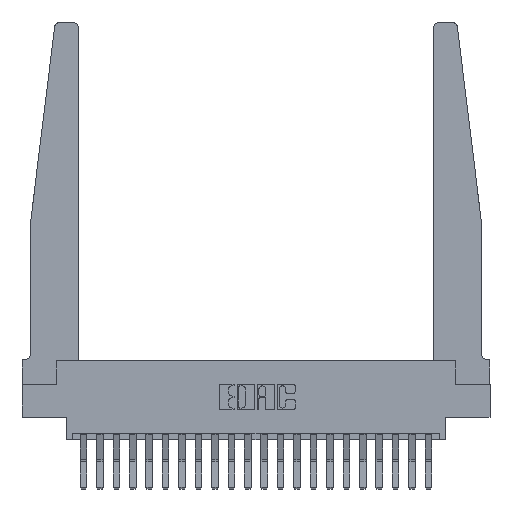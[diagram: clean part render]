
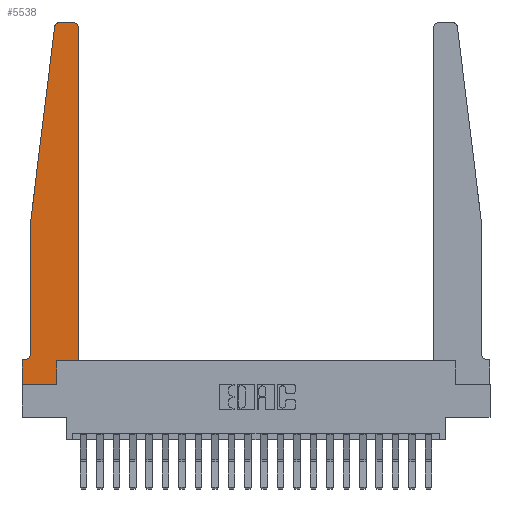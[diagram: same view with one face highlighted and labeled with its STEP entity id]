
A CAD part, top view. The second image highlights one B-rep face of the part: STEP entity #5538.
In plain terms, the highlighted planar face has unit normal (0, 0, 1).
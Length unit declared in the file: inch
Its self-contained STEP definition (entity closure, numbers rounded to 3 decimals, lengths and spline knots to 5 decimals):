
#519 = LINE ( 'NONE', #19762, #15685 ) ;
#530 = ORIENTED_EDGE ( 'NONE', *, *, #11995, .T. ) ;
#1284 = CARTESIAN_POINT ( 'NONE',  ( 0.015, 0.1875, 0.37 ) ) ;
#1354 = CARTESIAN_POINT ( 'NONE',  ( 0.2605, 0.18, 0.37 ) ) ;
#1542 = FACE_OUTER_BOUND ( 'NONE', #7784, .T. ) ;
#1668 = VECTOR ( 'NONE', #7958, 39.37008 ) ;
#2110 = EDGE_CURVE ( 'NONE', #18178, #5615, #8906, .T. ) ;
#2288 = CARTESIAN_POINT ( 'NONE',  ( 0.25, 2.75, 0.37 ) ) ;
#2576 = CARTESIAN_POINT ( 'NONE',  ( 0.065, 1.25, 0.37 ) ) ;
#3065 = VERTEX_POINT ( 'NONE', #1284 ) ;
#3131 = ORIENTED_EDGE ( 'NONE', *, *, #13566, .T. ) ;
#3146 = VERTEX_POINT ( 'NONE', #20632 ) ;
#3793 = CARTESIAN_POINT ( 'NONE',  ( 0.425, 0.18, 0.37 ) ) ;
#4312 = AXIS2_PLACEMENT_3D ( 'NONE', #20913, #17504, #19206 ) ;
#4415 = DIRECTION ( 'NONE',  ( 1., 0., 0. ) ) ;
#4659 = AXIS2_PLACEMENT_3D ( 'NONE', #18894, #22300, #20714 ) ;
#5538 = ADVANCED_FACE ( 'NONE', ( #1542 ), #15524, .T. ) ;
#5615 = VERTEX_POINT ( 'NONE', #15753 ) ;
#5729 = VECTOR ( 'NONE', #21569, 39.37008 ) ;
#6540 = EDGE_CURVE ( 'NONE', #12583, #21930, #21710, .T. ) ;
#6736 = EDGE_CURVE ( 'NONE', #16841, #12583, #519, .T. ) ;
#7322 = LINE ( 'NONE', #3793, #15606 ) ;
#7554 = DIRECTION ( 'NONE',  ( -1., 0., 0. ) ) ;
#7690 = CARTESIAN_POINT ( 'NONE',  ( 0.2605, 0.18, 0.37 ) ) ;
#7784 = EDGE_LOOP ( 'NONE', ( #19887, #14361, #12147, #13457, #8397, #8300, #14306, #13143, #3131, #13134, #18057, #530 ) ) ;
#7958 = DIRECTION ( 'NONE',  ( -1., 0., 0. ) ) ;
#8097 = VECTOR ( 'NONE', #10315, 39.37008 ) ;
#8300 = ORIENTED_EDGE ( 'NONE', *, *, #10617, .T. ) ;
#8338 = CARTESIAN_POINT ( 'NONE',  ( 0.425, 2.72, 0.37 ) ) ;
#8397 = ORIENTED_EDGE ( 'NONE', *, *, #13122, .T. ) ;
#8530 = VERTEX_POINT ( 'NONE', #7690 ) ;
#8849 = DIRECTION ( 'NONE',  ( 0., -1., 0. ) ) ;
#8906 = LINE ( 'NONE', #2288, #14376 ) ;
#8945 = CARTESIAN_POINT ( 'NONE',  ( 0.2605, 0., 0.37 ) ) ;
#9074 = CIRCLE ( 'NONE', #19403, 0.05 ) ;
#9170 = CARTESIAN_POINT ( 'NONE',  ( 0., 0., 0.37 ) ) ;
#9228 = EDGE_CURVE ( 'NONE', #5615, #21931, #14462, .T. ) ;
#9879 = CARTESIAN_POINT ( 'NONE',  ( 0.065, 0.1875, 0.37 ) ) ;
#10016 = LINE ( 'NONE', #1354, #18084 ) ;
#10315 = DIRECTION ( 'NONE',  ( 0., -1., 0. ) ) ;
#10617 = EDGE_CURVE ( 'NONE', #3065, #16841, #18864, .T. ) ;
#11229 = EDGE_CURVE ( 'NONE', #8530, #3146, #7322, .T. ) ;
#11834 = CARTESIAN_POINT ( 'NONE',  ( 0.395, 2.75, 0.37 ) ) ;
#11995 = EDGE_CURVE ( 'NONE', #20736, #18178, #14829, .T. ) ;
#12012 = DIRECTION ( 'NONE',  ( 1., 0., 0. ) ) ;
#12147 = ORIENTED_EDGE ( 'NONE', *, *, #14173, .T. ) ;
#12235 = CARTESIAN_POINT ( 'NONE',  ( 0., 0.1875, 0.37 ) ) ;
#12583 = VERTEX_POINT ( 'NONE', #9170 ) ;
#12765 = DIRECTION ( 'NONE',  ( -1., 0., 0. ) ) ;
#13122 = EDGE_CURVE ( 'NONE', #20722, #3065, #9074, .T. ) ;
#13134 = ORIENTED_EDGE ( 'NONE', *, *, #11229, .T. ) ;
#13143 = ORIENTED_EDGE ( 'NONE', *, *, #6540, .T. ) ;
#13457 = ORIENTED_EDGE ( 'NONE', *, *, #21767, .T. ) ;
#13566 = EDGE_CURVE ( 'NONE', #21930, #8530, #10016, .T. ) ;
#14173 = EDGE_CURVE ( 'NONE', #21931, #15163, #21679, .T. ) ;
#14306 = ORIENTED_EDGE ( 'NONE', *, *, #6736, .T. ) ;
#14361 = ORIENTED_EDGE ( 'NONE', *, *, #9228, .T. ) ;
#14376 = VECTOR ( 'NONE', #12765, 39.37008 ) ;
#14462 = CIRCLE ( 'NONE', #4659, 0.03 ) ;
#14829 = CIRCLE ( 'NONE', #4312, 0.03 ) ;
#15163 = VERTEX_POINT ( 'NONE', #18630 ) ;
#15324 = DIRECTION ( 'NONE',  ( 0., 1., 0. ) ) ;
#15524 = PLANE ( 'NONE',  #18808 ) ;
#15606 = VECTOR ( 'NONE', #19489, 39.37008 ) ;
#15685 = VECTOR ( 'NONE', #8849, 39.37008 ) ;
#15753 = CARTESIAN_POINT ( 'NONE',  ( 0.27653, 2.75, 0.37 ) ) ;
#16294 = DIRECTION ( 'NONE',  ( 0., 0., -1. ) ) ;
#16775 = CARTESIAN_POINT ( 'NONE',  ( 0., 0.1875, 0.37 ) ) ;
#16841 = VERTEX_POINT ( 'NONE', #16775 ) ;
#16916 = CARTESIAN_POINT ( 'NONE',  ( 0.425, 0.18, 0.37 ) ) ;
#16921 = CARTESIAN_POINT ( 'NONE',  ( 0., 0., 0.37 ) ) ;
#17090 = CARTESIAN_POINT ( 'NONE',  ( 0.065, 0.2375, 0.37 ) ) ;
#17359 = DIRECTION ( 'NONE',  ( 0., 0., 1. ) ) ;
#17504 = DIRECTION ( 'NONE',  ( 0., 0., 1. ) ) ;
#18057 = ORIENTED_EDGE ( 'NONE', *, *, #21023, .T. ) ;
#18084 = VECTOR ( 'NONE', #20597, 39.37008 ) ;
#18174 = LINE ( 'NONE', #2576, #8097 ) ;
#18178 = VERTEX_POINT ( 'NONE', #11834 ) ;
#18421 = CARTESIAN_POINT ( 'NONE',  ( 0.015, 0.2375, 0.37 ) ) ;
#18630 = CARTESIAN_POINT ( 'NONE',  ( 0.065, 1.25, 0.37 ) ) ;
#18808 = AXIS2_PLACEMENT_3D ( 'NONE', #12235, #17359, #12012 ) ;
#18864 = LINE ( 'NONE', #9879, #1668 ) ;
#18894 = CARTESIAN_POINT ( 'NONE',  ( 0.27653, 2.72, 0.37 ) ) ;
#19206 = DIRECTION ( 'NONE',  ( 1., 0., 0. ) ) ;
#19403 = AXIS2_PLACEMENT_3D ( 'NONE', #18421, #16294, #7554 ) ;
#19489 = DIRECTION ( 'NONE',  ( 1., 0., 0. ) ) ;
#19644 = CARTESIAN_POINT ( 'NONE',  ( 0.065, 1.25, 0.37 ) ) ;
#19694 = VECTOR ( 'NONE', #15324, 39.37008 ) ;
#19762 = CARTESIAN_POINT ( 'NONE',  ( 0., 0., 0.37 ) ) ;
#19887 = ORIENTED_EDGE ( 'NONE', *, *, #2110, .T. ) ;
#20597 = DIRECTION ( 'NONE',  ( 0., 1., 0. ) ) ;
#20632 = CARTESIAN_POINT ( 'NONE',  ( 0.425, 0.18, 0.37 ) ) ;
#20714 = DIRECTION ( 'NONE',  ( 1., 0., 0. ) ) ;
#20722 = VERTEX_POINT ( 'NONE', #17090 ) ;
#20736 = VERTEX_POINT ( 'NONE', #8338 ) ;
#20913 = CARTESIAN_POINT ( 'NONE',  ( 0.395, 2.72, 0.37 ) ) ;
#20986 = CARTESIAN_POINT ( 'NONE',  ( 0.24675, 2.72367, 0.37 ) ) ;
#21023 = EDGE_CURVE ( 'NONE', #3146, #20736, #22141, .T. ) ;
#21569 = DIRECTION ( 'NONE',  ( -0.122, -0.992, 0. ) ) ;
#21679 = LINE ( 'NONE', #19644, #5729 ) ;
#21710 = LINE ( 'NONE', #16921, #21832 ) ;
#21767 = EDGE_CURVE ( 'NONE', #15163, #20722, #18174, .T. ) ;
#21832 = VECTOR ( 'NONE', #4415, 39.37008 ) ;
#21930 = VERTEX_POINT ( 'NONE', #8945 ) ;
#21931 = VERTEX_POINT ( 'NONE', #20986 ) ;
#22141 = LINE ( 'NONE', #16916, #19694 ) ;
#22300 = DIRECTION ( 'NONE',  ( 0., 0., 1. ) ) ;
